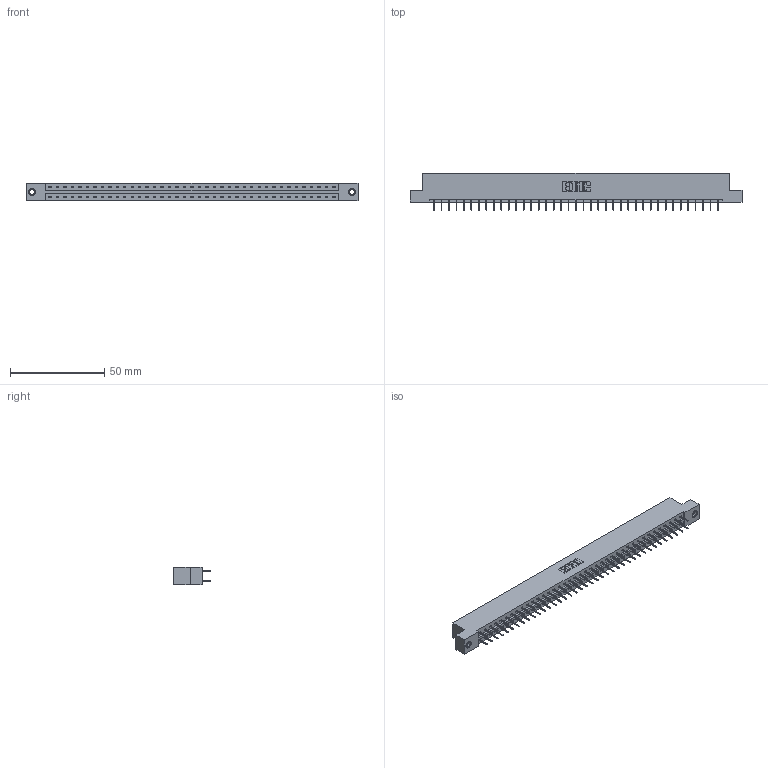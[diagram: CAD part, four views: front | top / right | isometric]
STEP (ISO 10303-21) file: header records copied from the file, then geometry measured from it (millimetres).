
FILE_DESCRIPTION (( 'STEP AP203' ), '1' );
FILE_NAME ('833-078-524-207.STEP', '2020-06-05T19:52:42', ( '' ), ( '' ), 'SwSTEP 2.0', 'SolidWorks 2020', '' );
FILE_SCHEMA (( 'CONFIG_CONTROL_DESIGN' ));
Length unit declared in the file: inch
Products named in the file (4): 833-078-524-207; 345-250-001_345-250-005-103; 345-292-001_345-293-124; 833 Part_Flush - .156 Dia - TI
Assembly tree (81 placements, depth 2):
  833-078-524-207
    833 Part_Flush - .156 Dia - TI
    345-292-001_345-293-124  x78
    345-250-001_345-250-005-103  x2
Bounding box: 176.07 x 19.69 x 9.4 mm (x, y, z)
Volume: 17816.4 mm3; surface area: 20711.1 mm2
Topology: 81 solids, 81 shells, 4542 faces, 12849 edges, 8246 vertices
Faces by surface type: plane 3378, cylinder 1148, cone 12, torus 4
Entity records: 26738 total; most frequent: CARTESIAN_POINT 4417, ORIENTED_EDGE 4346, DIRECTION 3811, EDGE_CURVE 2173, VECTOR 2029, LINE 2029, VERTEX_POINT 1440, AXIS2_PLACEMENT_3D 891
